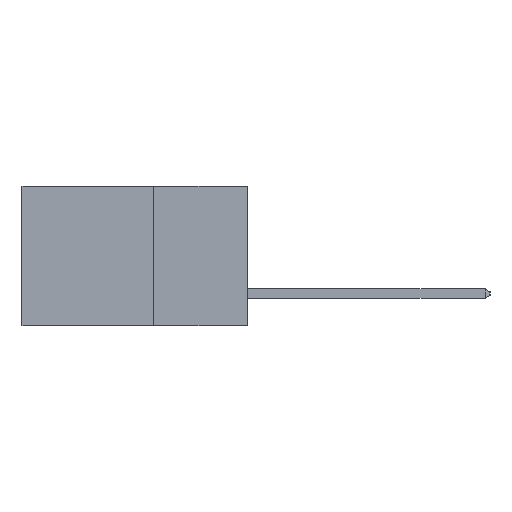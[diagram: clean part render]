
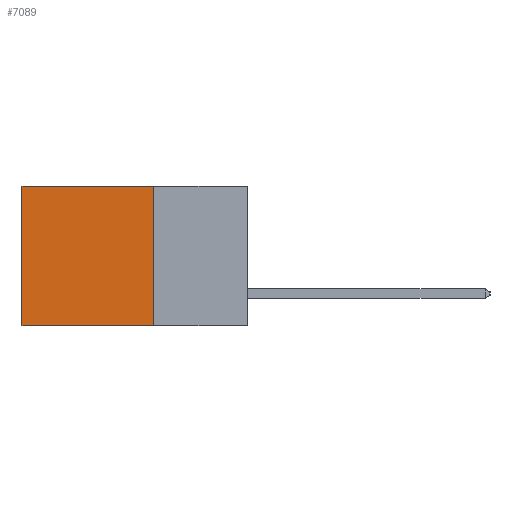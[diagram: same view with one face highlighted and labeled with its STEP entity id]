
A CAD part, left-side view. The second image highlights one B-rep face of the part: STEP entity #7089.
In plain terms, the highlighted planar face has unit normal (-1, 0, 0).
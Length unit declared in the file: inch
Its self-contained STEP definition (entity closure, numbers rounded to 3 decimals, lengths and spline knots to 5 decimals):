
#28 = ORIENTED_EDGE ( 'NONE', *, *, #6402, .T. ) ;
#594 = EDGE_CURVE ( 'NONE', #6093, #7548, #10500, .T. ) ;
#700 = DIRECTION ( 'NONE',  ( 0., 1., 0. ) ) ;
#738 = CARTESIAN_POINT ( 'NONE',  ( 0.2615, 0.25, -0.37 ) ) ;
#887 = LINE ( 'NONE', #9120, #3422 ) ;
#1618 = CARTESIAN_POINT ( 'NONE',  ( 0.2615, 0.6, -0.37 ) ) ;
#1795 = CARTESIAN_POINT ( 'NONE',  ( 0.2615, 0.25, -0.37 ) ) ;
#1826 = DIRECTION ( 'NONE',  ( 0., 0., -1. ) ) ;
#2061 = ORIENTED_EDGE ( 'NONE', *, *, #5783, .T. ) ;
#2453 = VERTEX_POINT ( 'NONE', #11291 ) ;
#2488 = CARTESIAN_POINT ( 'NONE',  ( 0.2615, 0.25, -0.37 ) ) ;
#2924 = CARTESIAN_POINT ( 'NONE',  ( 0.2615, 0.25, 0. ) ) ;
#3327 = EDGE_LOOP ( 'NONE', ( #2061, #6738, #3552, #28 ) ) ;
#3422 = VECTOR ( 'NONE', #700, 39.37008 ) ;
#3552 = ORIENTED_EDGE ( 'NONE', *, *, #594, .F. ) ;
#3976 = DIRECTION ( 'NONE',  ( 0., 1., 0. ) ) ;
#4037 = CARTESIAN_POINT ( 'NONE',  ( 0.2615, 0.6, -0.37 ) ) ;
#4440 = EDGE_CURVE ( 'NONE', #7548, #12801, #887, .T. ) ;
#5783 = EDGE_CURVE ( 'NONE', #2453, #12801, #9232, .T. ) ;
#6093 = VERTEX_POINT ( 'NONE', #11653 ) ;
#6402 = EDGE_CURVE ( 'NONE', #6093, #2453, #6892, .T. ) ;
#6738 = ORIENTED_EDGE ( 'NONE', *, *, #4440, .F. ) ;
#6892 = LINE ( 'NONE', #2924, #9627 ) ;
#7089 = ADVANCED_FACE ( 'NONE', ( #12710 ), #12093, .F. ) ;
#7193 = DIRECTION ( 'NONE',  ( 0., 0., -1. ) ) ;
#7548 = VERTEX_POINT ( 'NONE', #2488 ) ;
#8129 = DIRECTION ( 'NONE',  ( 1., 0., 0. ) ) ;
#9120 = CARTESIAN_POINT ( 'NONE',  ( 0.2615, 0.25, -0.37 ) ) ;
#9232 = LINE ( 'NONE', #4037, #11572 ) ;
#9627 = VECTOR ( 'NONE', #3976, 39.37008 ) ;
#10500 = LINE ( 'NONE', #1795, #12485 ) ;
#11291 = CARTESIAN_POINT ( 'NONE',  ( 0.2615, 0.6, 0. ) ) ;
#11572 = VECTOR ( 'NONE', #7193, 39.37008 ) ;
#11653 = CARTESIAN_POINT ( 'NONE',  ( 0.2615, 0.25, 0. ) ) ;
#11973 = AXIS2_PLACEMENT_3D ( 'NONE', #738, #8129, #1826 ) ;
#12093 = PLANE ( 'NONE',  #11973 ) ;
#12485 = VECTOR ( 'NONE', #12855, 39.37008 ) ;
#12710 = FACE_OUTER_BOUND ( 'NONE', #3327, .T. ) ;
#12801 = VERTEX_POINT ( 'NONE', #1618 ) ;
#12855 = DIRECTION ( 'NONE',  ( 0., 0., -1. ) ) ;
